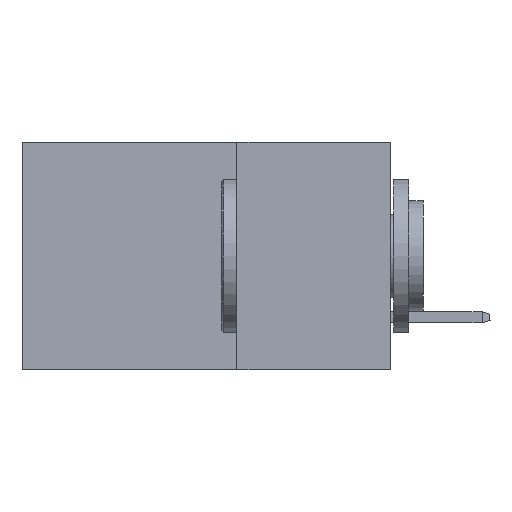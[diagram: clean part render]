
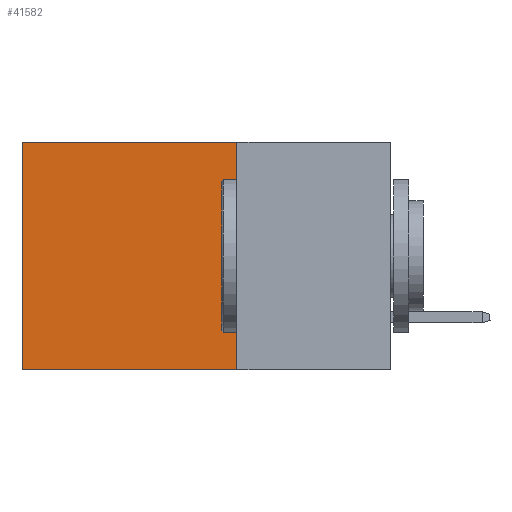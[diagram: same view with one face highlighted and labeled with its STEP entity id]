
A CAD part, left-side view. The second image highlights one B-rep face of the part: STEP entity #41582.
In plain terms, the highlighted planar face has unit normal (-1, 0, 0).
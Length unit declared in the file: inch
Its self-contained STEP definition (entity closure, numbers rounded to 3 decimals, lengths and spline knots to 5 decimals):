
#932 = DIRECTION ( 'NONE',  ( 0., 1., 0. ) ) ;
#2154 = VECTOR ( 'NONE', #10919, 39.37008 ) ;
#3657 = ORIENTED_EDGE ( 'NONE', *, *, #24041, .F. ) ;
#4132 = LINE ( 'NONE', #10995, #29098 ) ;
#7185 = EDGE_LOOP ( 'NONE', ( #28823, #3657, #27649, #22940 ) ) ;
#7861 = VECTOR ( 'NONE', #34429, 39.37008 ) ;
#9541 = LINE ( 'NONE', #26794, #2154 ) ;
#9643 = DIRECTION ( 'NONE',  ( 0., 1., 0. ) ) ;
#10919 = DIRECTION ( 'NONE',  ( 0., 0., -1. ) ) ;
#10995 = CARTESIAN_POINT ( 'NONE',  ( 0.2875, 0.25, 0. ) ) ;
#13832 = FACE_OUTER_BOUND ( 'NONE', #7185, .T. ) ;
#14425 = VERTEX_POINT ( 'NONE', #18563 ) ;
#15404 = VERTEX_POINT ( 'NONE', #39079 ) ;
#16839 = DIRECTION ( 'NONE',  ( 0., 0., -1. ) ) ;
#17407 = EDGE_CURVE ( 'NONE', #14425, #37854, #4132, .T. ) ;
#18563 = CARTESIAN_POINT ( 'NONE',  ( 0.2875, 0.25, 0. ) ) ;
#18689 = LINE ( 'NONE', #39980, #33590 ) ;
#22940 = ORIENTED_EDGE ( 'NONE', *, *, #17407, .T. ) ;
#23944 = DIRECTION ( 'NONE',  ( 1., 0., 0. ) ) ;
#24041 = EDGE_CURVE ( 'NONE', #30367, #15404, #18689, .T. ) ;
#25078 = EDGE_CURVE ( 'NONE', #37854, #15404, #9541, .T. ) ;
#26794 = CARTESIAN_POINT ( 'NONE',  ( 0.2875, 0.6, 0. ) ) ;
#27194 = PLANE ( 'NONE',  #43437 ) ;
#27649 = ORIENTED_EDGE ( 'NONE', *, *, #28856, .F. ) ;
#28823 = ORIENTED_EDGE ( 'NONE', *, *, #25078, .T. ) ;
#28856 = EDGE_CURVE ( 'NONE', #14425, #30367, #35571, .T. ) ;
#29098 = VECTOR ( 'NONE', #932, 39.37008 ) ;
#30367 = VERTEX_POINT ( 'NONE', #33282 ) ;
#30515 = CARTESIAN_POINT ( 'NONE',  ( 0.2875, 0.25, 0. ) ) ;
#30772 = CARTESIAN_POINT ( 'NONE',  ( 0.2875, 0.6, 0. ) ) ;
#31131 = CARTESIAN_POINT ( 'NONE',  ( 0.2875, 0.25, 0. ) ) ;
#33282 = CARTESIAN_POINT ( 'NONE',  ( 0.2875, 0.25, -0.37 ) ) ;
#33590 = VECTOR ( 'NONE', #9643, 39.37008 ) ;
#34429 = DIRECTION ( 'NONE',  ( 0., 0., -1. ) ) ;
#35571 = LINE ( 'NONE', #31131, #7861 ) ;
#37854 = VERTEX_POINT ( 'NONE', #30772 ) ;
#39079 = CARTESIAN_POINT ( 'NONE',  ( 0.2875, 0.6, -0.37 ) ) ;
#39980 = CARTESIAN_POINT ( 'NONE',  ( 0.2875, 0.25, -0.37 ) ) ;
#41582 = ADVANCED_FACE ( 'NONE', ( #13832 ), #27194, .F. ) ;
#43437 = AXIS2_PLACEMENT_3D ( 'NONE', #30515, #23944, #16839 ) ;
